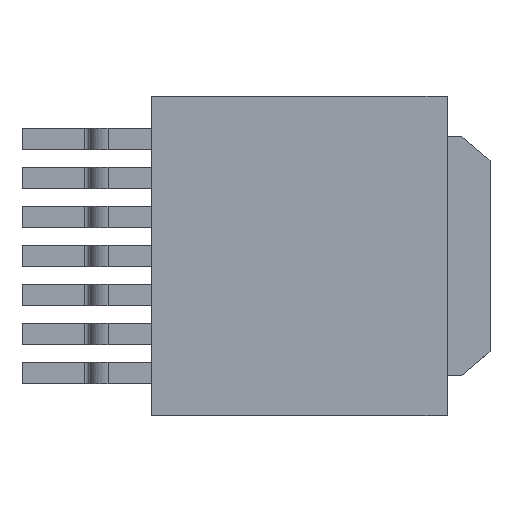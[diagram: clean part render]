
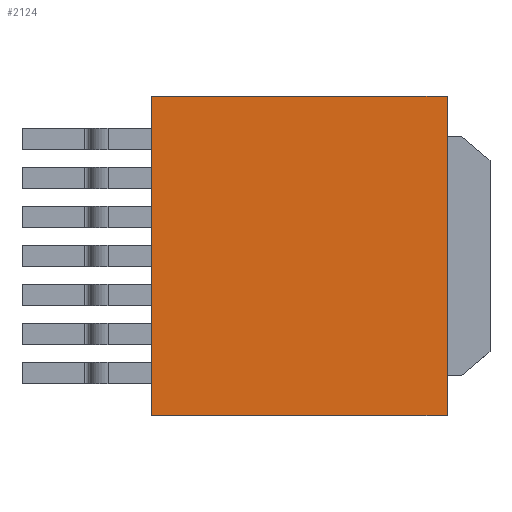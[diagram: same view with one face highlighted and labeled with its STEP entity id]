
A CAD part, top view. The second image highlights one B-rep face of the part: STEP entity #2124.
In plain terms, the highlighted planar face has unit normal (0, 0, 1).
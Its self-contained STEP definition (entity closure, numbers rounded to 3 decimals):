
#205=FACE_OUTER_BOUND('',#310,.T.);
#310=EDGE_LOOP('',(#1790,#1791,#1792,#1793));
#546=LINE('',#3420,#778);
#547=LINE('',#3422,#779);
#548=LINE('',#3424,#780);
#549=LINE('',#3425,#781);
#778=VECTOR('',#2832,1.);
#779=VECTOR('',#2833,1.);
#780=VECTOR('',#2834,1.);
#781=VECTOR('',#2835,1.);
#974=VERTEX_POINT('',#3418);
#975=VERTEX_POINT('',#3419);
#976=VERTEX_POINT('',#3421);
#977=VERTEX_POINT('',#3423);
#1258=EDGE_CURVE('',#974,#975,#546,.T.);
#1259=EDGE_CURVE('',#975,#976,#547,.T.);
#1260=EDGE_CURVE('',#976,#977,#548,.T.);
#1261=EDGE_CURVE('',#977,#974,#549,.T.);
#1790=ORIENTED_EDGE('',*,*,#1258,.T.);
#1791=ORIENTED_EDGE('',*,*,#1259,.T.);
#1792=ORIENTED_EDGE('',*,*,#1260,.T.);
#1793=ORIENTED_EDGE('',*,*,#1261,.T.);
#1914=PLANE('',#2287);
#2124=ADVANCED_FACE('',(#205),#1914,.T.);
#2287=AXIS2_PLACEMENT_3D('',#3417,#2830,#2831);
#2830=DIRECTION('center_axis',(0.,0.,1.));
#2831=DIRECTION('ref_axis',(-1.,0.,0.));
#2832=DIRECTION('',(0.,-1.,0.));
#2833=DIRECTION('',(1.,0.,0.));
#2834=DIRECTION('',(0.,1.,0.));
#2835=DIRECTION('',(-1.,0.,0.));
#3417=CARTESIAN_POINT('Origin',(2.81,0.,4.7));
#3418=CARTESIAN_POINT('',(-2.005,5.2,4.7));
#3419=CARTESIAN_POINT('',(-2.005,-5.2,4.7));
#3420=CARTESIAN_POINT('',(-2.005,0.,4.7));
#3421=CARTESIAN_POINT('',(7.625,-5.2,4.7));
#3422=CARTESIAN_POINT('',(2.81,-5.2,4.7));
#3423=CARTESIAN_POINT('',(7.625,5.2,4.7));
#3424=CARTESIAN_POINT('',(7.625,0.,4.7));
#3425=CARTESIAN_POINT('',(2.81,5.2,4.7));
